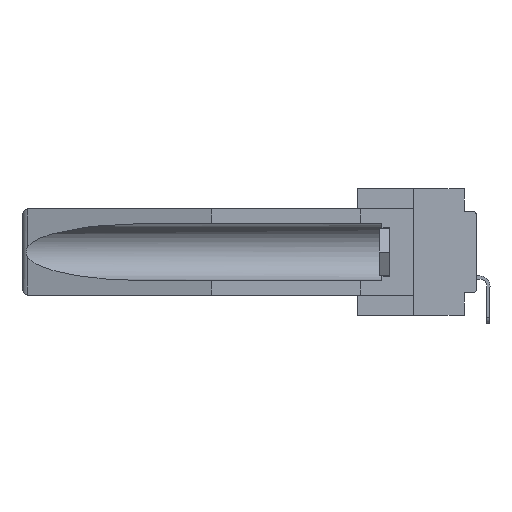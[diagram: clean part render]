
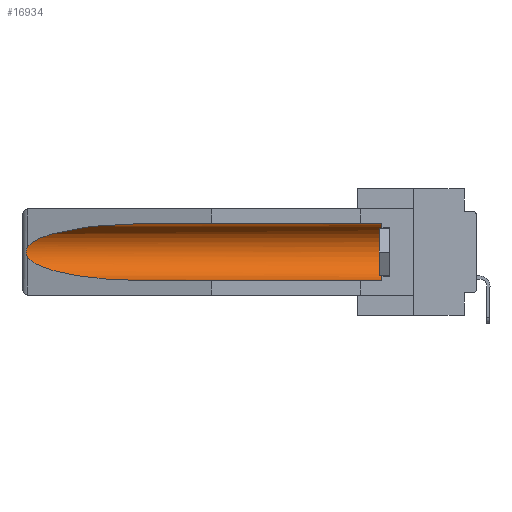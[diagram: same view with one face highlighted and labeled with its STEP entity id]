
A CAD part, left-side view. The second image highlights one B-rep face of the part: STEP entity #16934.
In plain terms, the highlighted cylindrical face has radius 2.857 mm (diameter 5.715 mm), a partial arc.
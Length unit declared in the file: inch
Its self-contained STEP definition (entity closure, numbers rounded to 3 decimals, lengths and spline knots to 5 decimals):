
#227 = VERTEX_POINT ( 'NONE', #16831 ) ;
#931 = EDGE_LOOP ( 'NONE', ( #18050, #31328, #5066, #5590, #1244, #10824 ) ) ;
#1052 = EDGE_CURVE ( 'NONE', #227, #18116, #26908, .T. ) ;
#1244 = ORIENTED_EDGE ( 'NONE', *, *, #24717, .T. ) ;
#1341 = DIRECTION ( 'NONE',  ( 0., 1., 0. ) ) ;
#1585 = CARTESIAN_POINT ( 'NONE',  ( 0.26537, 1.52718, -0.19328 ) ) ;
#2604 = CARTESIAN_POINT ( 'NONE',  ( 0.21114, 1.30732, -0.284 ) ) ;
#4407 = CARTESIAN_POINT ( 'NONE',  ( 0.155, 1.07973, -0.059 ) ) ;
#4474 = DIRECTION ( 'NONE',  ( 0., 0., 1. ) ) ;
#4748 = VERTEX_POINT ( 'NONE', #31707 ) ;
#5066 = ORIENTED_EDGE ( 'NONE', *, *, #34529, .T. ) ;
#5590 = ORIENTED_EDGE ( 'NONE', *, *, #23762, .F. ) ;
#5596 = CARTESIAN_POINT ( 'NONE',  ( 0.155, 0.126, -0.1715 ) ) ;
#8177 = DIRECTION ( 'NONE',  ( 0., -1., 0. ) ) ;
#8564 = CARTESIAN_POINT ( 'NONE',  ( 0.155, 0.126, -0.059 ) ) ;
#8665 = VERTEX_POINT ( 'NONE', #23839 ) ;
#9063 = CARTESIAN_POINT ( 'NONE',  ( 0.155, -0.30754, -0.284 ) ) ;
#9073 = VERTEX_POINT ( 'NONE', #8564 ) ;
#9166 = B_SPLINE_CURVE_WITH_KNOTS ( 'NONE', 3,
 ( #15142, #34425, #15487, #23658, #23425, #15374, #12904, #9961, #29037, #1585 ),
 .UNSPECIFIED., .F., .F.,
 ( 4, 2, 2, 2, 4 ),
 ( 0., 0.00029, 0.00058, 0.00087, 0.00117 ),
 .UNSPECIFIED. ) ;
#9961 = CARTESIAN_POINT ( 'NONE',  ( 0.26655, 1.53094, -0.18657 ) ) ;
#10041 = CYLINDRICAL_SURFACE ( 'NONE', #10508, 0.1125 ) ;
#10378 = VERTEX_POINT ( 'NONE', #20691 ) ;
#10508 = AXIS2_PLACEMENT_3D ( 'NONE', #15301, #17904, #4474 ) ;
#10824 = ORIENTED_EDGE ( 'NONE', *, *, #22044, .T. ) ;
#11200 = VECTOR ( 'NONE', #27685, 39.37008 ) ;
#12603 = VECTOR ( 'NONE', #1341, 39.37008 ) ;
#12904 = CARTESIAN_POINT ( 'NONE',  ( 0.2673, 1.53269, -0.17917 ) ) ;
#15016 = CARTESIAN_POINT ( 'NONE',  ( 0.26537, 1.52718, -0.14972 ) ) ;
#15142 = CARTESIAN_POINT ( 'NONE',  ( 0.26537, 1.52718, -0.14972 ) ) ;
#15301 = CARTESIAN_POINT ( 'NONE',  ( 0.155, -0.30754, -0.1715 ) ) ;
#15374 = CARTESIAN_POINT ( 'NONE',  ( 0.2675, 1.53308, -0.17534 ) ) ;
#15487 = CARTESIAN_POINT ( 'NONE',  ( 0.26654, 1.53092, -0.15636 ) ) ;
#16831 = CARTESIAN_POINT ( 'NONE',  ( 0.155, 1.07973, -0.059 ) ) ;
#16934 = ADVANCED_FACE ( 'NONE', ( #25678 ), #10041, .F. ) ;
#17904 = DIRECTION ( 'NONE',  ( 0., 1., 0. ) ) ;
#18050 = ORIENTED_EDGE ( 'NONE', *, *, #1052, .T. ) ;
#18116 = VERTEX_POINT ( 'NONE', #28206 ) ;
#18386 = LINE ( 'NONE', #9063, #11200 ) ;
#18544 = CARTESIAN_POINT ( 'NONE',  ( 0.25451, 1.48313, -0.24835 ) ) ;
#20691 = CARTESIAN_POINT ( 'NONE',  ( 0.26537, 1.52718, -0.19328 ) ) ;
#22044 = EDGE_CURVE ( 'NONE', #9073, #227, #34078, .T. ) ;
#22141 = EDGE_CURVE ( 'NONE', #18116, #10378, #9166, .T. ) ;
#23425 = CARTESIAN_POINT ( 'NONE',  ( 0.2675, 1.53308, -0.16763 ) ) ;
#23449 =( BOUNDED_CURVE ( )  B_SPLINE_CURVE ( 3, ( #26675, #18544, #2604, #29021 ),
 .UNSPECIFIED., .F., .F. ) 
 B_SPLINE_CURVE_WITH_KNOTS ( ( 4, 4 ),
 ( 0.1948, 1.5708 ),
 .UNSPECIFIED. ) 
 CURVE ( )  GEOMETRIC_REPRESENTATION_ITEM ( )  RATIONAL_B_SPLINE_CURVE ( ( 1., 0.848, 0.848, 1. ) ) 
 REPRESENTATION_ITEM ( '' )  );
#23658 = CARTESIAN_POINT ( 'NONE',  ( 0.2673, 1.5327, -0.16383 ) ) ;
#23762 = EDGE_CURVE ( 'NONE', #8665, #4748, #18386, .T. ) ;
#23839 = CARTESIAN_POINT ( 'NONE',  ( 0.155, 0.126, -0.284 ) ) ;
#24257 = AXIS2_PLACEMENT_3D ( 'NONE', #5596, #8177, #29710 ) ;
#24717 = EDGE_CURVE ( 'NONE', #8665, #9073, #31679, .T. ) ;
#25678 = FACE_OUTER_BOUND ( 'NONE', #931, .T. ) ;
#25759 = CARTESIAN_POINT ( 'NONE',  ( 0.21114, 1.30732, -0.059 ) ) ;
#26675 = CARTESIAN_POINT ( 'NONE',  ( 0.26537, 1.52718, -0.19328 ) ) ;
#26908 =( BOUNDED_CURVE ( )  B_SPLINE_CURVE ( 3, ( #4407, #25759, #28225, #15016 ),
 .UNSPECIFIED., .F., .F. ) 
 B_SPLINE_CURVE_WITH_KNOTS ( ( 4, 4 ),
 ( 4.71239, 6.08839 ),
 .UNSPECIFIED. ) 
 CURVE ( )  GEOMETRIC_REPRESENTATION_ITEM ( )  RATIONAL_B_SPLINE_CURVE ( ( 1., 0.848, 0.848, 1. ) ) 
 REPRESENTATION_ITEM ( '' )  );
#27685 = DIRECTION ( 'NONE',  ( 0., 1., 0. ) ) ;
#28206 = CARTESIAN_POINT ( 'NONE',  ( 0.26537, 1.52718, -0.14972 ) ) ;
#28225 = CARTESIAN_POINT ( 'NONE',  ( 0.25451, 1.48313, -0.09465 ) ) ;
#28351 = CARTESIAN_POINT ( 'NONE',  ( 0.155, -0.30754, -0.059 ) ) ;
#29021 = CARTESIAN_POINT ( 'NONE',  ( 0.155, 1.07973, -0.284 ) ) ;
#29037 = CARTESIAN_POINT ( 'NONE',  ( 0.26597, 1.5296, -0.19026 ) ) ;
#29710 = DIRECTION ( 'NONE',  ( 0., 0., 1. ) ) ;
#31328 = ORIENTED_EDGE ( 'NONE', *, *, #22141, .T. ) ;
#31679 = CIRCLE ( 'NONE', #24257, 0.1125 ) ;
#31707 = CARTESIAN_POINT ( 'NONE',  ( 0.155, 1.07973, -0.284 ) ) ;
#34078 = LINE ( 'NONE', #28351, #12603 ) ;
#34425 = CARTESIAN_POINT ( 'NONE',  ( 0.26597, 1.52961, -0.15275 ) ) ;
#34529 = EDGE_CURVE ( 'NONE', #10378, #4748, #23449, .T. ) ;
